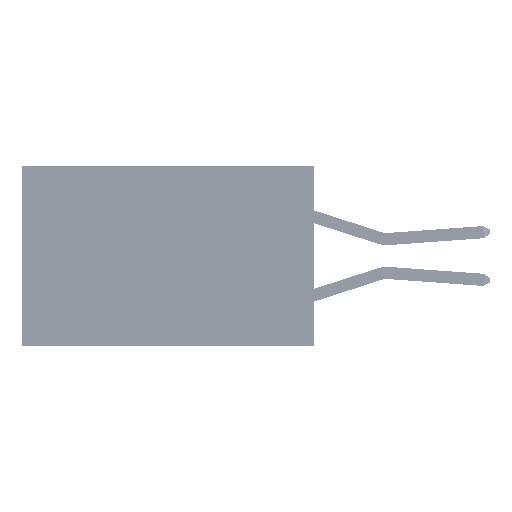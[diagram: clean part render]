
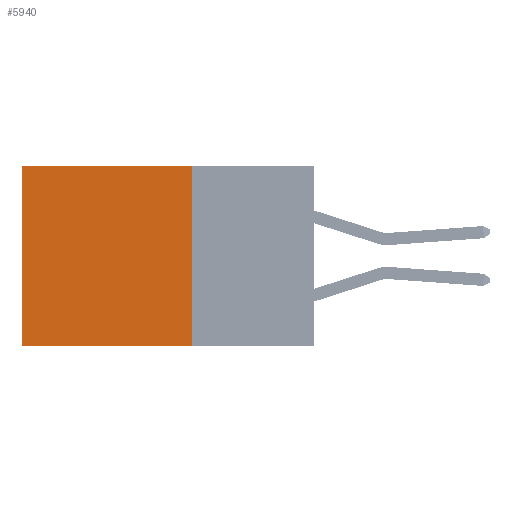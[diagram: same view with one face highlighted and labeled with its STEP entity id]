
A CAD part, left-side view. The second image highlights one B-rep face of the part: STEP entity #5940.
In plain terms, the highlighted planar face has unit normal (-1, 0, 0).
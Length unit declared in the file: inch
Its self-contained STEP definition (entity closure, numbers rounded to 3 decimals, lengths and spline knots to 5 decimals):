
#564 = CARTESIAN_POINT ( 'NONE',  ( 0.2875, 0.6, -0.37 ) ) ;
#2236 = FACE_OUTER_BOUND ( 'NONE', #38675, .T. ) ;
#5940 = ADVANCED_FACE ( 'NONE', ( #2236 ), #12249, .F. ) ;
#6657 = CARTESIAN_POINT ( 'NONE',  ( 0.2875, 0.6, 0. ) ) ;
#7900 = LINE ( 'NONE', #9418, #32662 ) ;
#8219 = CARTESIAN_POINT ( 'NONE',  ( 0.2875, 0.25, 0. ) ) ;
#8792 = VERTEX_POINT ( 'NONE', #6657 ) ;
#8919 = DIRECTION ( 'NONE',  ( 0., 0., -1. ) ) ;
#9023 = VERTEX_POINT ( 'NONE', #45961 ) ;
#9418 = CARTESIAN_POINT ( 'NONE',  ( 0.2875, 0.6, 0. ) ) ;
#10046 = EDGE_CURVE ( 'NONE', #8792, #45675, #7900, .T. ) ;
#12249 = PLANE ( 'NONE',  #44891 ) ;
#14351 = CARTESIAN_POINT ( 'NONE',  ( 0.2875, 0.25, -0.37 ) ) ;
#15379 = DIRECTION ( 'NONE',  ( 0., 1., 0. ) ) ;
#16735 = DIRECTION ( 'NONE',  ( 0., 0., -1. ) ) ;
#17153 = DIRECTION ( 'NONE',  ( 0., 0., -1. ) ) ;
#17820 = EDGE_CURVE ( 'NONE', #9023, #45675, #48736, .T. ) ;
#21679 = DIRECTION ( 'NONE',  ( 0., 1., 0. ) ) ;
#23247 = VERTEX_POINT ( 'NONE', #37580 ) ;
#23865 = EDGE_CURVE ( 'NONE', #23247, #8792, #24764, .T. ) ;
#24764 = LINE ( 'NONE', #46134, #36242 ) ;
#25180 = VECTOR ( 'NONE', #16735, 39.37008 ) ;
#28323 = ORIENTED_EDGE ( 'NONE', *, *, #17820, .F. ) ;
#29992 = EDGE_CURVE ( 'NONE', #23247, #9023, #31289, .T. ) ;
#31289 = LINE ( 'NONE', #40213, #25180 ) ;
#32662 = VECTOR ( 'NONE', #8919, 39.37008 ) ;
#32754 = ORIENTED_EDGE ( 'NONE', *, *, #10046, .T. ) ;
#36242 = VECTOR ( 'NONE', #15379, 39.37008 ) ;
#37291 = VECTOR ( 'NONE', #21679, 39.37008 ) ;
#37580 = CARTESIAN_POINT ( 'NONE',  ( 0.2875, 0.25, 0. ) ) ;
#38675 = EDGE_LOOP ( 'NONE', ( #32754, #28323, #49555, #46683 ) ) ;
#39269 = DIRECTION ( 'NONE',  ( 1., 0., 0. ) ) ;
#40213 = CARTESIAN_POINT ( 'NONE',  ( 0.2875, 0.25, 0. ) ) ;
#44891 = AXIS2_PLACEMENT_3D ( 'NONE', #8219, #39269, #17153 ) ;
#45675 = VERTEX_POINT ( 'NONE', #564 ) ;
#45961 = CARTESIAN_POINT ( 'NONE',  ( 0.2875, 0.25, -0.37 ) ) ;
#46134 = CARTESIAN_POINT ( 'NONE',  ( 0.2875, 0.25, 0. ) ) ;
#46683 = ORIENTED_EDGE ( 'NONE', *, *, #23865, .T. ) ;
#48736 = LINE ( 'NONE', #14351, #37291 ) ;
#49555 = ORIENTED_EDGE ( 'NONE', *, *, #29992, .F. ) ;
